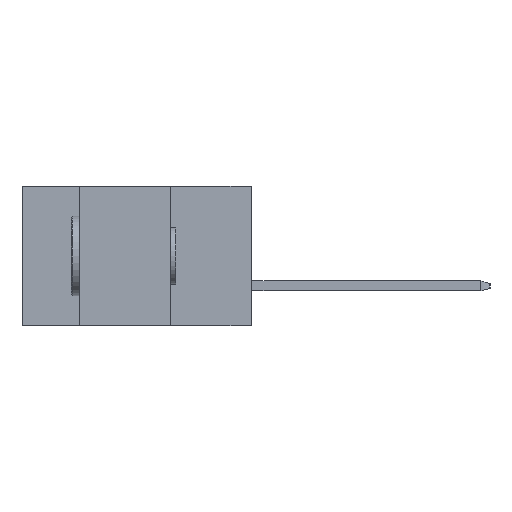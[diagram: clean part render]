
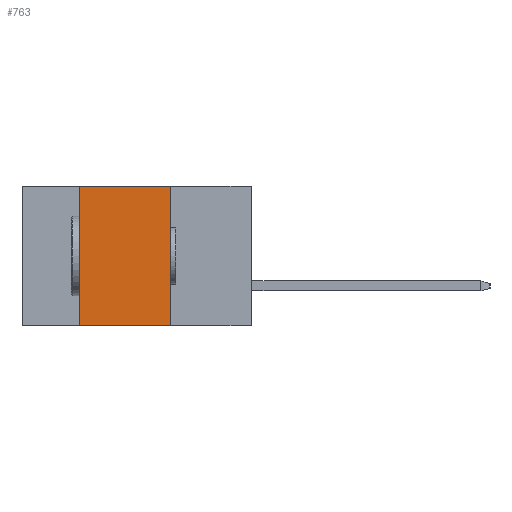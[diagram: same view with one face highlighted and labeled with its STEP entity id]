
A CAD part, left-side view. The second image highlights one B-rep face of the part: STEP entity #763.
In plain terms, the highlighted planar face has unit normal (-1, 0, 0).
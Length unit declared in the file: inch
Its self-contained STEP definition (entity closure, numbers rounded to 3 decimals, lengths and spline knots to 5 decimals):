
#209 = VECTOR ( 'NONE', #7057, 39.37008 ) ;
#233 = CARTESIAN_POINT ( 'NONE',  ( 0., 0.72, -0.437 ) ) ;
#620 = VERTEX_POINT ( 'NONE', #5112 ) ;
#649 = CARTESIAN_POINT ( 'NONE',  ( 0., 0.72, 0. ) ) ;
#763 = ADVANCED_FACE ( 'NONE', ( #5820 ), #9507, .F. ) ;
#1150 = CARTESIAN_POINT ( 'NONE',  ( 0., 0.54, -0.437 ) ) ;
#1179 = ORIENTED_EDGE ( 'NONE', *, *, #3404, .F. ) ;
#1377 = CARTESIAN_POINT ( 'NONE',  ( 0., 0.54, 0. ) ) ;
#1462 = ORIENTED_EDGE ( 'NONE', *, *, #5397, .F. ) ;
#2150 = DIRECTION ( 'NONE',  ( 1., 0., 0. ) ) ;
#2216 = AXIS2_PLACEMENT_3D ( 'NONE', #9407, #2150, #7895 ) ;
#2660 = EDGE_CURVE ( 'NONE', #6442, #6658, #9139, .T. ) ;
#3108 = VECTOR ( 'NONE', #7021, 39.37008 ) ;
#3404 = EDGE_CURVE ( 'NONE', #6658, #4063, #9569, .T. ) ;
#3646 = DIRECTION ( 'NONE',  ( 0., -1., 0. ) ) ;
#3683 = ORIENTED_EDGE ( 'NONE', *, *, #8650, .T. ) ;
#4063 = VERTEX_POINT ( 'NONE', #9593 ) ;
#5010 = VECTOR ( 'NONE', #3646, 39.37008 ) ;
#5112 = CARTESIAN_POINT ( 'NONE',  ( 0., 0.254, -0.437 ) ) ;
#5397 = EDGE_CURVE ( 'NONE', #4063, #620, #8367, .T. ) ;
#5467 = LINE ( 'NONE', #233, #3108 ) ;
#5473 = EDGE_LOOP ( 'NONE', ( #1462, #1179, #6468, #3683 ) ) ;
#5820 = FACE_OUTER_BOUND ( 'NONE', #5473, .T. ) ;
#6442 = VERTEX_POINT ( 'NONE', #8636 ) ;
#6468 = ORIENTED_EDGE ( 'NONE', *, *, #2660, .F. ) ;
#6658 = VERTEX_POINT ( 'NONE', #1377 ) ;
#6871 = CARTESIAN_POINT ( 'NONE',  ( 0., 0.254, -0.437 ) ) ;
#7021 = DIRECTION ( 'NONE',  ( 0., -1., 0. ) ) ;
#7057 = DIRECTION ( 'NONE',  ( 0., 0., 1. ) ) ;
#7685 = DIRECTION ( 'NONE',  ( 0., 0., -1. ) ) ;
#7895 = DIRECTION ( 'NONE',  ( 0., 0., -1. ) ) ;
#8367 = LINE ( 'NONE', #6871, #8480 ) ;
#8480 = VECTOR ( 'NONE', #7685, 39.37008 ) ;
#8636 = CARTESIAN_POINT ( 'NONE',  ( 0., 0.54, -0.437 ) ) ;
#8650 = EDGE_CURVE ( 'NONE', #6442, #620, #5467, .T. ) ;
#9139 = LINE ( 'NONE', #1150, #209 ) ;
#9407 = CARTESIAN_POINT ( 'NONE',  ( 0., 0.72, 0. ) ) ;
#9507 = PLANE ( 'NONE',  #2216 ) ;
#9569 = LINE ( 'NONE', #649, #5010 ) ;
#9593 = CARTESIAN_POINT ( 'NONE',  ( 0., 0.254, 0. ) ) ;
